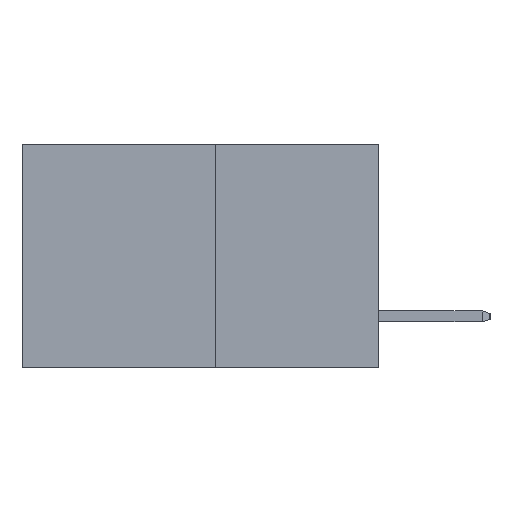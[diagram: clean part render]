
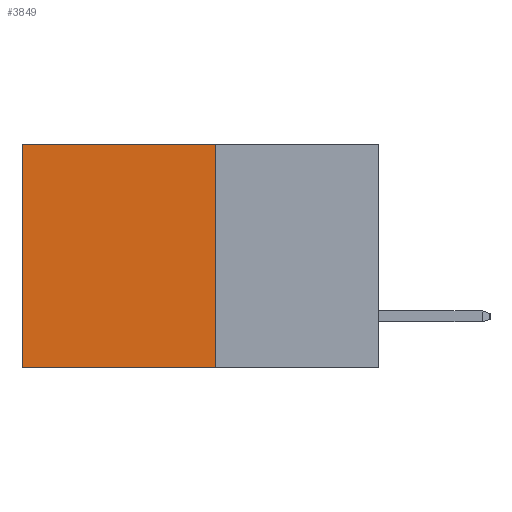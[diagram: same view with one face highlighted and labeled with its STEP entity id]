
A CAD part, left-side view. The second image highlights one B-rep face of the part: STEP entity #3849.
In plain terms, the highlighted planar face has unit normal (-1, 0, 0).
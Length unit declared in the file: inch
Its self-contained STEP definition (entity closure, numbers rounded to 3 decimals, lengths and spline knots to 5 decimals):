
#109 = FACE_OUTER_BOUND ( 'NONE', #2951, .T. ) ;
#172 = CARTESIAN_POINT ( 'NONE',  ( 0.277, 0.27, -0.37 ) ) ;
#297 = LINE ( 'NONE', #7064, #6894 ) ;
#573 = DIRECTION ( 'NONE',  ( 1., 0., 0. ) ) ;
#654 = PLANE ( 'NONE',  #4777 ) ;
#696 = VERTEX_POINT ( 'NONE', #829 ) ;
#712 = DIRECTION ( 'NONE',  ( 0., 0., -1. ) ) ;
#829 = CARTESIAN_POINT ( 'NONE',  ( 0.277, 0.27, 0. ) ) ;
#844 = CARTESIAN_POINT ( 'NONE',  ( 0.277, 0.27, -0.37 ) ) ;
#1147 = ORIENTED_EDGE ( 'NONE', *, *, #6849, .F. ) ;
#2829 = LINE ( 'NONE', #5816, #9167 ) ;
#2951 = EDGE_LOOP ( 'NONE', ( #5537, #7634, #1147, #5784 ) ) ;
#3084 = EDGE_CURVE ( 'NONE', #696, #9983, #10032, .T. ) ;
#3318 = CARTESIAN_POINT ( 'NONE',  ( 0.277, 0.59, -0.37 ) ) ;
#3849 = ADVANCED_FACE ( 'NONE', ( #109 ), #654, .F. ) ;
#3878 = VECTOR ( 'NONE', #10399, 39.37008 ) ;
#4167 = EDGE_CURVE ( 'NONE', #9983, #8437, #2829, .T. ) ;
#4777 = AXIS2_PLACEMENT_3D ( 'NONE', #844, #573, #712 ) ;
#4808 = LINE ( 'NONE', #9918, #8772 ) ;
#5276 = VERTEX_POINT ( 'NONE', #172 ) ;
#5537 = ORIENTED_EDGE ( 'NONE', *, *, #4167, .T. ) ;
#5784 = ORIENTED_EDGE ( 'NONE', *, *, #3084, .T. ) ;
#5816 = CARTESIAN_POINT ( 'NONE',  ( 0.277, 0.59, -0.37 ) ) ;
#5845 = DIRECTION ( 'NONE',  ( 0., 0., -1. ) ) ;
#6066 = EDGE_CURVE ( 'NONE', #5276, #8437, #4808, .T. ) ;
#6849 = EDGE_CURVE ( 'NONE', #696, #5276, #297, .T. ) ;
#6894 = VECTOR ( 'NONE', #8303, 39.37008 ) ;
#7064 = CARTESIAN_POINT ( 'NONE',  ( 0.277, 0.27, -0.37 ) ) ;
#7634 = ORIENTED_EDGE ( 'NONE', *, *, #6066, .F. ) ;
#8303 = DIRECTION ( 'NONE',  ( 0., 0., -1. ) ) ;
#8437 = VERTEX_POINT ( 'NONE', #3318 ) ;
#8772 = VECTOR ( 'NONE', #9907, 39.37008 ) ;
#9167 = VECTOR ( 'NONE', #5845, 39.37008 ) ;
#9907 = DIRECTION ( 'NONE',  ( 0., 1., 0. ) ) ;
#9918 = CARTESIAN_POINT ( 'NONE',  ( 0.277, 0.27, -0.37 ) ) ;
#9983 = VERTEX_POINT ( 'NONE', #10466 ) ;
#10032 = LINE ( 'NONE', #10419, #3878 ) ;
#10399 = DIRECTION ( 'NONE',  ( 0., 1., 0. ) ) ;
#10419 = CARTESIAN_POINT ( 'NONE',  ( 0.277, 0.27, 0. ) ) ;
#10466 = CARTESIAN_POINT ( 'NONE',  ( 0.277, 0.59, 0. ) ) ;
